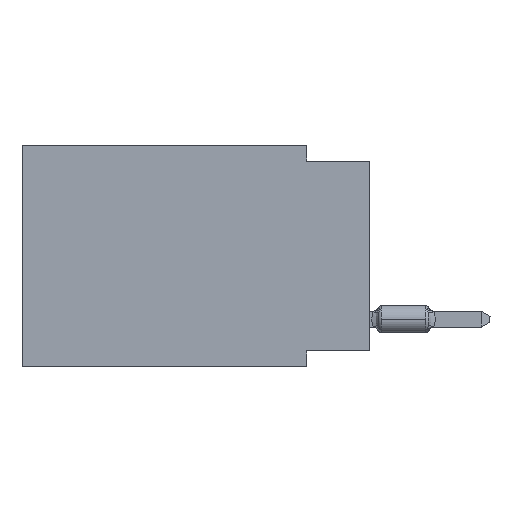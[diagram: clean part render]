
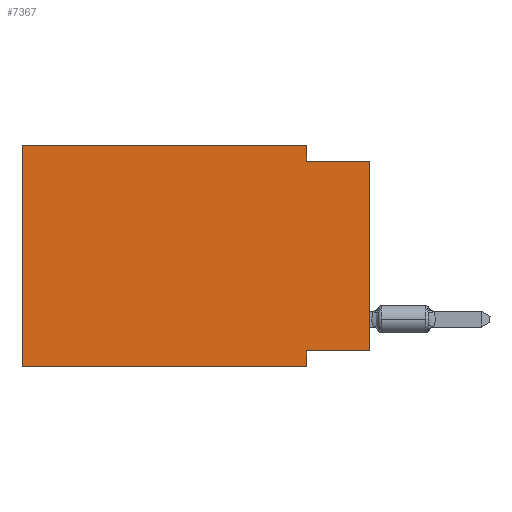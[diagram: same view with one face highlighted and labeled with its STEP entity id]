
A CAD part, left-side view. The second image highlights one B-rep face of the part: STEP entity #7367.
In plain terms, the highlighted planar face has unit normal (-1, 0, 0).
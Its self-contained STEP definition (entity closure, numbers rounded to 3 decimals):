
#455 = LINE ( 'NONE', #45293, #46475 ) ;
#664 = ORIENTED_EDGE ( 'NONE', *, *, #45514, .F. ) ;
#676 = DIRECTION ( 'NONE',  ( 0., -1., 0. ) ) ;
#1318 = DIRECTION ( 'NONE',  ( 0., -1., 0. ) ) ;
#2012 = EDGE_CURVE ( 'NONE', #30800, #9833, #34930, .T. ) ;
#2105 = DIRECTION ( 'NONE',  ( 0., 0., -1. ) ) ;
#2293 = ORIENTED_EDGE ( 'NONE', *, *, #26959, .T. ) ;
#2657 = CARTESIAN_POINT ( 'NONE',  ( 0., 13.97, 0. ) ) ;
#2721 = CARTESIAN_POINT ( 'NONE',  ( 0., 13.97, -8.89 ) ) ;
#6876 = DIRECTION ( 'NONE',  ( 0., 0., 1. ) ) ;
#6991 = AXIS2_PLACEMENT_3D ( 'NONE', #2657, #29270, #2105 ) ;
#7020 = PLANE ( 'NONE',  #6991 ) ;
#7367 = ADVANCED_FACE ( 'NONE', ( #41729 ), #7020, .F. ) ;
#9833 = VERTEX_POINT ( 'NONE', #31191 ) ;
#12493 = DIRECTION ( 'NONE',  ( 0., 0., -1. ) ) ;
#15260 = VERTEX_POINT ( 'NONE', #44694 ) ;
#15289 = EDGE_CURVE ( 'NONE', #21002, #53863, #23281, .T. ) ;
#15650 = EDGE_CURVE ( 'NONE', #32557, #15260, #35365, .T. ) ;
#18485 = EDGE_CURVE ( 'NONE', #9833, #21002, #20758, .T. ) ;
#20758 = LINE ( 'NONE', #25379, #33617 ) ;
#21002 = VERTEX_POINT ( 'NONE', #34712 ) ;
#21573 = VECTOR ( 'NONE', #676, 1000. ) ;
#21913 = ORIENTED_EDGE ( 'NONE', *, *, #18485, .F. ) ;
#22709 = DIRECTION ( 'NONE',  ( 0., 0., -1. ) ) ;
#22742 = VECTOR ( 'NONE', #6876, 1000. ) ;
#23281 = LINE ( 'NONE', #35439, #39909 ) ;
#25379 = CARTESIAN_POINT ( 'NONE',  ( 0., 13.97, 0. ) ) ;
#26816 = DIRECTION ( 'NONE',  ( 0., 0., 1. ) ) ;
#26959 = EDGE_CURVE ( 'NONE', #30800, #37559, #455, .T. ) ;
#27538 = DIRECTION ( 'NONE',  ( 0., 1., 0. ) ) ;
#27583 = CARTESIAN_POINT ( 'NONE',  ( 0., 0., -0.635 ) ) ;
#28475 = EDGE_CURVE ( 'NONE', #53863, #36352, #49567, .T. ) ;
#28584 = ORIENTED_EDGE ( 'NONE', *, *, #28475, .F. ) ;
#29270 = DIRECTION ( 'NONE',  ( 1., 0., 0. ) ) ;
#30634 = ORIENTED_EDGE ( 'NONE', *, *, #15650, .F. ) ;
#30800 = VERTEX_POINT ( 'NONE', #2721 ) ;
#31191 = CARTESIAN_POINT ( 'NONE',  ( 0., 13.97, 0. ) ) ;
#31255 = CARTESIAN_POINT ( 'NONE',  ( 0., 2.54, -8.89 ) ) ;
#31429 = EDGE_CURVE ( 'NONE', #32557, #36352, #42431, .T. ) ;
#32513 = CARTESIAN_POINT ( 'NONE',  ( 0., 2.54, -0.635 ) ) ;
#32557 = VERTEX_POINT ( 'NONE', #35625 ) ;
#32731 = VECTOR ( 'NONE', #12493, 1000. ) ;
#33617 = VECTOR ( 'NONE', #38396, 1000. ) ;
#34039 = CARTESIAN_POINT ( 'NONE',  ( 0., 0., -0.635 ) ) ;
#34712 = CARTESIAN_POINT ( 'NONE',  ( 0., 2.54, 0. ) ) ;
#34930 = LINE ( 'NONE', #48528, #55881 ) ;
#35168 = ORIENTED_EDGE ( 'NONE', *, *, #2012, .F. ) ;
#35365 = LINE ( 'NONE', #35935, #38899 ) ;
#35439 = CARTESIAN_POINT ( 'NONE',  ( 0., 2.54, 0. ) ) ;
#35625 = CARTESIAN_POINT ( 'NONE',  ( 0., 0., -8.255 ) ) ;
#35935 = CARTESIAN_POINT ( 'NONE',  ( 0., 0., -8.255 ) ) ;
#36352 = VERTEX_POINT ( 'NONE', #34039 ) ;
#36784 = EDGE_LOOP ( 'NONE', ( #44617, #28584, #41541, #21913, #35168, #2293, #664, #30634 ) ) ;
#37559 = VERTEX_POINT ( 'NONE', #40720 ) ;
#38094 = CARTESIAN_POINT ( 'NONE',  ( 0., 0., 0. ) ) ;
#38396 = DIRECTION ( 'NONE',  ( 0., -1., 0. ) ) ;
#38899 = VECTOR ( 'NONE', #27538, 1000. ) ;
#39371 = LINE ( 'NONE', #31255, #32731 ) ;
#39909 = VECTOR ( 'NONE', #22709, 1000. ) ;
#40720 = CARTESIAN_POINT ( 'NONE',  ( 0., 2.54, -8.89 ) ) ;
#41541 = ORIENTED_EDGE ( 'NONE', *, *, #15289, .F. ) ;
#41729 = FACE_OUTER_BOUND ( 'NONE', #36784, .T. ) ;
#42431 = LINE ( 'NONE', #38094, #22742 ) ;
#44617 = ORIENTED_EDGE ( 'NONE', *, *, #31429, .T. ) ;
#44694 = CARTESIAN_POINT ( 'NONE',  ( 0., 2.54, -8.255 ) ) ;
#45293 = CARTESIAN_POINT ( 'NONE',  ( 0., 13.97, -8.89 ) ) ;
#45514 = EDGE_CURVE ( 'NONE', #15260, #37559, #39371, .T. ) ;
#46475 = VECTOR ( 'NONE', #1318, 1000. ) ;
#48528 = CARTESIAN_POINT ( 'NONE',  ( 0., 13.97, 0. ) ) ;
#49567 = LINE ( 'NONE', #27583, #21573 ) ;
#53863 = VERTEX_POINT ( 'NONE', #32513 ) ;
#55881 = VECTOR ( 'NONE', #26816, 1000. ) ;
